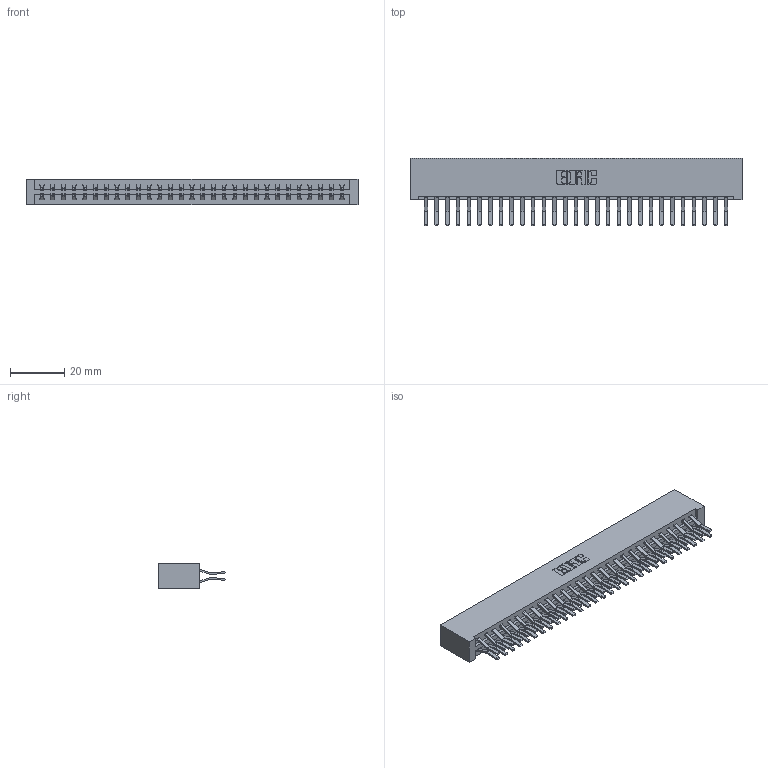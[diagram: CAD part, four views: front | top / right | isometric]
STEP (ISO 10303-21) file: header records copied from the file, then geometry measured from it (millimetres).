
FILE_DESCRIPTION (( 'STEP AP203' ), '1' );
FILE_NAME ('387-058-560-201.STEP', '2018-09-21T02:27:25', ( '' ), ( '' ), 'SwSTEP 2.0', 'SolidWorks 2016', '' );
FILE_SCHEMA (( 'CONFIG_CONTROL_DESIGN' ));
Length unit declared in the file: inch
Products named in the file (3): 345-292-001_560 Tail; 387-058-560-201; 337 Part_No Mounting Lugs
Assembly tree (59 placements, depth 2):
  387-058-560-201
    337 Part_No Mounting Lugs
    345-292-001_560 Tail  x58
Bounding box: 122.78 x 24.78 x 9.4 mm (x, y, z)
Volume: 13907.8 mm3; surface area: 16752.9 mm2
Topology: 59 solids, 59 shells, 3354 faces, 9973 edges, 6570 vertices
Faces by surface type: plane 2270, cylinder 1084
Entity records: 23977 total; most frequent: CARTESIAN_POINT 4050, ORIENTED_EDGE 3986, DIRECTION 3465, EDGE_CURVE 1993, LINE 1869, VECTOR 1869, VERTEX_POINT 1326, AXIS2_PLACEMENT_3D 798
